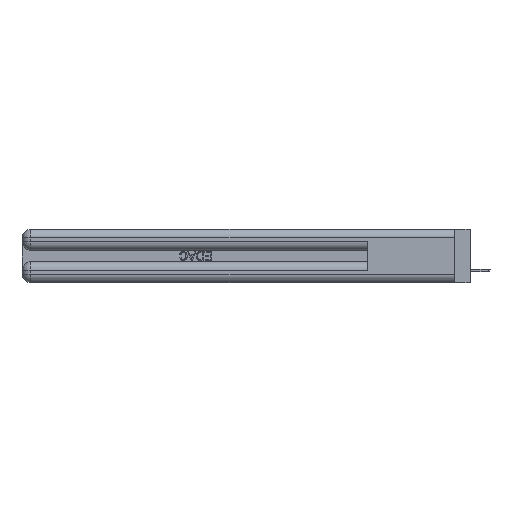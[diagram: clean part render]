
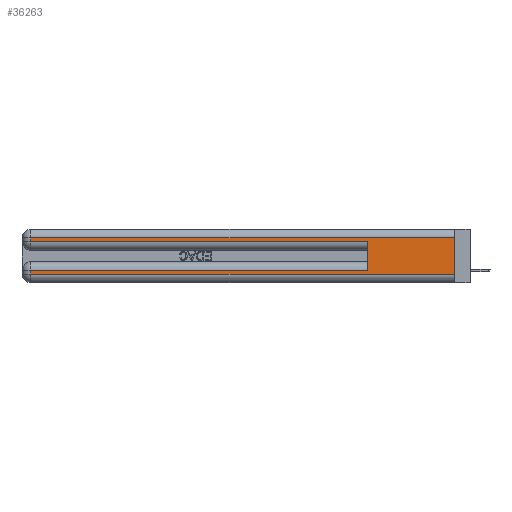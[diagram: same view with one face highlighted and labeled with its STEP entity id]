
A CAD part, left-side view. The second image highlights one B-rep face of the part: STEP entity #36263.
In plain terms, the highlighted planar face has unit normal (-1, 0, 0).
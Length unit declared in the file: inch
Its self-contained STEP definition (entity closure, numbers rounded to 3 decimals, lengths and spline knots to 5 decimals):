
#718 = VECTOR ( 'NONE', #16957, 39.37008 ) ;
#2042 = CARTESIAN_POINT ( 'NONE',  ( 0., 0., 0.31 ) ) ;
#2130 = CARTESIAN_POINT ( 'NONE',  ( 0., 2.94, 0.085 ) ) ;
#3231 = VECTOR ( 'NONE', #22242, 39.37008 ) ;
#4854 = VERTEX_POINT ( 'NONE', #39076 ) ;
#4945 = EDGE_CURVE ( 'NONE', #18595, #24584, #15602, .T. ) ;
#5680 = CARTESIAN_POINT ( 'NONE',  ( 0., 0.6, 0.085 ) ) ;
#5836 = CARTESIAN_POINT ( 'NONE',  ( 0., 0.6, 0.285 ) ) ;
#6437 = LINE ( 'NONE', #16644, #24203 ) ;
#6659 = VERTEX_POINT ( 'NONE', #2042 ) ;
#11619 = ORIENTED_EDGE ( 'NONE', *, *, #15142, .T. ) ;
#12052 = CARTESIAN_POINT ( 'NONE',  ( 0., 2.94, 0.37 ) ) ;
#12115 = VERTEX_POINT ( 'NONE', #19086 ) ;
#13562 = VERTEX_POINT ( 'NONE', #5836 ) ;
#14003 = CARTESIAN_POINT ( 'NONE',  ( 0., 2.94, 0.31 ) ) ;
#14423 = ORIENTED_EDGE ( 'NONE', *, *, #23716, .F. ) ;
#15142 = EDGE_CURVE ( 'NONE', #12115, #13562, #25527, .T. ) ;
#15602 = LINE ( 'NONE', #12052, #3231 ) ;
#15862 = EDGE_CURVE ( 'NONE', #6659, #38874, #40529, .T. ) ;
#16644 = CARTESIAN_POINT ( 'NONE',  ( 0., 0., 0.06 ) ) ;
#16934 = DIRECTION ( 'NONE',  ( 0., 0., 1. ) ) ;
#16957 = DIRECTION ( 'NONE',  ( 0., 0., -1. ) ) ;
#18272 = CARTESIAN_POINT ( 'NONE',  ( 0., 2.94, 0.37 ) ) ;
#18283 = ORIENTED_EDGE ( 'NONE', *, *, #41029, .F. ) ;
#18594 = EDGE_LOOP ( 'NONE', ( #18283, #36447, #35570, #11619, #14423, #34195, #31472, #28072 ) ) ;
#18595 = VERTEX_POINT ( 'NONE', #2130 ) ;
#18751 = CARTESIAN_POINT ( 'NONE',  ( 0., 2.94, 0.06 ) ) ;
#19086 = CARTESIAN_POINT ( 'NONE',  ( 0., 2.94, 0.285 ) ) ;
#19511 = DIRECTION ( 'NONE',  ( 0., 0., -1. ) ) ;
#19830 = PLANE ( 'NONE',  #40899 ) ;
#19875 = VERTEX_POINT ( 'NONE', #5680 ) ;
#22242 = DIRECTION ( 'NONE',  ( 0., 0., -1. ) ) ;
#23140 = FACE_OUTER_BOUND ( 'NONE', #18594, .T. ) ;
#23686 = CARTESIAN_POINT ( 'NONE',  ( 0., 0., 0.31 ) ) ;
#23716 = EDGE_CURVE ( 'NONE', #19875, #13562, #43511, .T. ) ;
#24078 = VECTOR ( 'NONE', #16934, 39.37008 ) ;
#24203 = VECTOR ( 'NONE', #30124, 39.37008 ) ;
#24584 = VERTEX_POINT ( 'NONE', #18751 ) ;
#25527 = LINE ( 'NONE', #31738, #42805 ) ;
#25718 = EDGE_CURVE ( 'NONE', #24584, #4854, #6437, .T. ) ;
#27216 = EDGE_CURVE ( 'NONE', #19875, #18595, #28796, .T. ) ;
#27361 = LINE ( 'NONE', #37561, #718 ) ;
#28072 = ORIENTED_EDGE ( 'NONE', *, *, #25718, .T. ) ;
#28644 = DIRECTION ( 'NONE',  ( 0., -1., 0. ) ) ;
#28796 = LINE ( 'NONE', #32336, #37052 ) ;
#30124 = DIRECTION ( 'NONE',  ( 0., -1., 0. ) ) ;
#31198 = DIRECTION ( 'NONE',  ( 0., 1., 0. ) ) ;
#31472 = ORIENTED_EDGE ( 'NONE', *, *, #4945, .T. ) ;
#31738 = CARTESIAN_POINT ( 'NONE',  ( 0., 0., 0.285 ) ) ;
#32336 = CARTESIAN_POINT ( 'NONE',  ( 0., 0., 0.085 ) ) ;
#34195 = ORIENTED_EDGE ( 'NONE', *, *, #27216, .T. ) ;
#34664 = DIRECTION ( 'NONE',  ( 1., 0., 0. ) ) ;
#35249 = DIRECTION ( 'NONE',  ( 0., 1., 0. ) ) ;
#35570 = ORIENTED_EDGE ( 'NONE', *, *, #41591, .T. ) ;
#36263 = ADVANCED_FACE ( 'NONE', ( #23140 ), #19830, .F. ) ;
#36447 = ORIENTED_EDGE ( 'NONE', *, *, #15862, .T. ) ;
#36493 = VECTOR ( 'NONE', #31198, 39.37008 ) ;
#37052 = VECTOR ( 'NONE', #35249, 39.37008 ) ;
#37561 = CARTESIAN_POINT ( 'NONE',  ( 0., 0., 0.37 ) ) ;
#38430 = LINE ( 'NONE', #18272, #41119 ) ;
#38874 = VERTEX_POINT ( 'NONE', #14003 ) ;
#39076 = CARTESIAN_POINT ( 'NONE',  ( 0., 0., 0.06 ) ) ;
#40415 = CARTESIAN_POINT ( 'NONE',  ( 0., 0.6, 0.145 ) ) ;
#40529 = LINE ( 'NONE', #23686, #36493 ) ;
#40654 = DIRECTION ( 'NONE',  ( 0., 0., -1. ) ) ;
#40878 = CARTESIAN_POINT ( 'NONE',  ( 0., 0., 0.37 ) ) ;
#40899 = AXIS2_PLACEMENT_3D ( 'NONE', #40878, #34664, #40654 ) ;
#41029 = EDGE_CURVE ( 'NONE', #6659, #4854, #27361, .T. ) ;
#41119 = VECTOR ( 'NONE', #19511, 39.37008 ) ;
#41591 = EDGE_CURVE ( 'NONE', #38874, #12115, #38430, .T. ) ;
#42805 = VECTOR ( 'NONE', #28644, 39.37008 ) ;
#43511 = LINE ( 'NONE', #40415, #24078 ) ;
